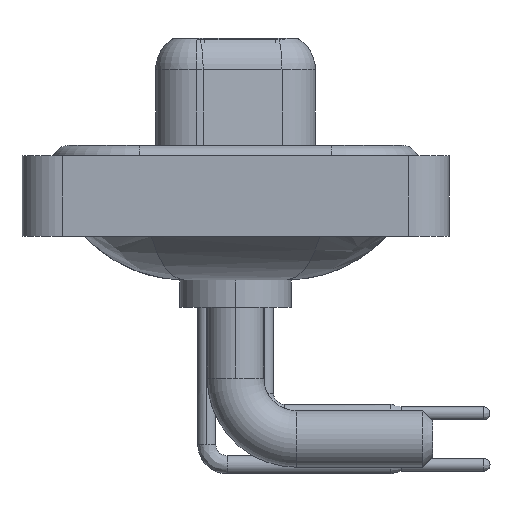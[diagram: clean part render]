
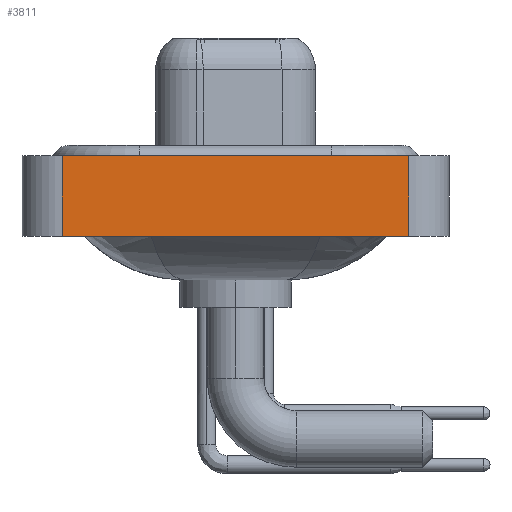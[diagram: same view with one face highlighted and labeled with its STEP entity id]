
A CAD part, left-side view. The second image highlights one B-rep face of the part: STEP entity #3811.
In plain terms, the highlighted planar face has unit normal (-1, 0, 0).
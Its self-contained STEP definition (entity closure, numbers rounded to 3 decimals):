
#1337 = EDGE_CURVE ( 'NONE', #9711, #18341, #13243, .T. ) ;
#2509 = DIRECTION ( 'NONE',  ( 0., 0., 1. ) ) ;
#3601 = ORIENTED_EDGE ( 'NONE', *, *, #8723, .T. ) ;
#3811 = ADVANCED_FACE ( 'NONE', ( #12301 ), #15376, .T. ) ;
#4435 = VECTOR ( 'NONE', #2509, 1000. ) ;
#6525 = VECTOR ( 'NONE', #14263, 1000. ) ;
#6567 = CARTESIAN_POINT ( 'NONE',  ( -7.35, 8.55, -3.6 ) ) ;
#7058 = VERTEX_POINT ( 'NONE', #9611 ) ;
#7788 = DIRECTION ( 'NONE',  ( 0., -1., 0. ) ) ;
#7899 = CARTESIAN_POINT ( 'NONE',  ( -7.35, -8.55, 0.4 ) ) ;
#8477 = CARTESIAN_POINT ( 'NONE',  ( -7.35, 8.55, 0.4 ) ) ;
#8723 = EDGE_CURVE ( 'NONE', #9711, #7058, #13087, .T. ) ;
#9014 = DIRECTION ( 'NONE',  ( 0., 0., 1. ) ) ;
#9192 = CARTESIAN_POINT ( 'NONE',  ( -7.35, -8.55, -3.6 ) ) ;
#9611 = CARTESIAN_POINT ( 'NONE',  ( -7.35, -8.55, -3.6 ) ) ;
#9711 = VERTEX_POINT ( 'NONE', #6567 ) ;
#10431 = CARTESIAN_POINT ( 'NONE',  ( -7.35, -8.55, 0.4 ) ) ;
#10769 = LINE ( 'NONE', #7899, #20123 ) ;
#11206 = VERTEX_POINT ( 'NONE', #10431 ) ;
#12301 = FACE_OUTER_BOUND ( 'NONE', #17499, .T. ) ;
#13087 = LINE ( 'NONE', #9192, #6525 ) ;
#13243 = LINE ( 'NONE', #14729, #15972 ) ;
#13847 = ORIENTED_EDGE ( 'NONE', *, *, #1337, .F. ) ;
#14075 = EDGE_CURVE ( 'NONE', #7058, #11206, #15052, .T. ) ;
#14263 = DIRECTION ( 'NONE',  ( 0., -1., 0. ) ) ;
#14729 = CARTESIAN_POINT ( 'NONE',  ( -7.35, 8.55, -3.6 ) ) ;
#15052 = LINE ( 'NONE', #15369, #4435 ) ;
#15369 = CARTESIAN_POINT ( 'NONE',  ( -7.35, -8.55, -3.6 ) ) ;
#15376 = PLANE ( 'NONE',  #17007 ) ;
#15822 = ORIENTED_EDGE ( 'NONE', *, *, #14075, .T. ) ;
#15972 = VECTOR ( 'NONE', #16536, 1000. ) ;
#16536 = DIRECTION ( 'NONE',  ( 0., 0., 1. ) ) ;
#17007 = AXIS2_PLACEMENT_3D ( 'NONE', #17150, #18856, #9014 ) ;
#17150 = CARTESIAN_POINT ( 'NONE',  ( -7.35, -8.55, -3.6 ) ) ;
#17499 = EDGE_LOOP ( 'NONE', ( #15822, #20398, #13847, #3601 ) ) ;
#17770 = EDGE_CURVE ( 'NONE', #18341, #11206, #10769, .T. ) ;
#18341 = VERTEX_POINT ( 'NONE', #8477 ) ;
#18856 = DIRECTION ( 'NONE',  ( -1., 0., 0. ) ) ;
#20123 = VECTOR ( 'NONE', #7788, 1000. ) ;
#20398 = ORIENTED_EDGE ( 'NONE', *, *, #17770, .F. ) ;
